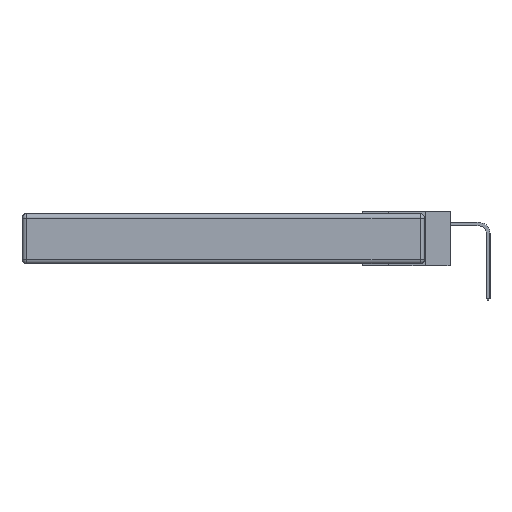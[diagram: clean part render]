
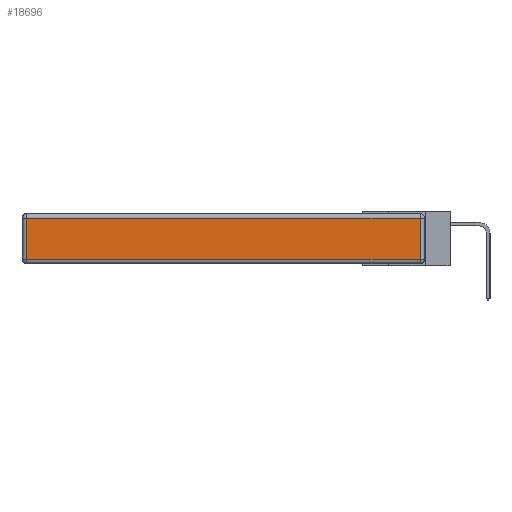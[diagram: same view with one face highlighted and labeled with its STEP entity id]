
A CAD part, left-side view. The second image highlights one B-rep face of the part: STEP entity #18696.
In plain terms, the highlighted planar face has unit normal (-1, 0, 0).
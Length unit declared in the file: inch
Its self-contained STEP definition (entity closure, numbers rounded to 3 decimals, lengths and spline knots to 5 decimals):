
#203 = DIRECTION ( 'NONE',  ( 0., 0., 1. ) ) ;
#385 = CARTESIAN_POINT ( 'NONE',  ( 0., 2.72, -0.343 ) ) ;
#1299 = CARTESIAN_POINT ( 'NONE',  ( 0., 0., -0.313 ) ) ;
#3633 = LINE ( 'NONE', #25424, #27488 ) ;
#4889 = LINE ( 'NONE', #385, #25835 ) ;
#6402 = EDGE_CURVE ( 'NONE', #10515, #11674, #4889, .T. ) ;
#6538 = EDGE_LOOP ( 'NONE', ( #11590, #15237, #15600, #9331 ) ) ;
#8997 = FACE_OUTER_BOUND ( 'NONE', #6538, .T. ) ;
#9331 = ORIENTED_EDGE ( 'NONE', *, *, #6402, .T. ) ;
#10515 = VERTEX_POINT ( 'NONE', #21889 ) ;
#11590 = ORIENTED_EDGE ( 'NONE', *, *, #17142, .T. ) ;
#11674 = VERTEX_POINT ( 'NONE', #11871 ) ;
#11871 = CARTESIAN_POINT ( 'NONE',  ( 0., 2.72, -0.313 ) ) ;
#13286 = CARTESIAN_POINT ( 'NONE',  ( 0., 0.03, -0.313 ) ) ;
#14312 = DIRECTION ( 'NONE',  ( -1., 0., 0. ) ) ;
#15237 = ORIENTED_EDGE ( 'NONE', *, *, #17485, .T. ) ;
#15278 = CARTESIAN_POINT ( 'NONE',  ( 0., 0.03, -0.03 ) ) ;
#15600 = ORIENTED_EDGE ( 'NONE', *, *, #19342, .T. ) ;
#15658 = VERTEX_POINT ( 'NONE', #13286 ) ;
#16502 = DIRECTION ( 'NONE',  ( 0., 0., 1. ) ) ;
#16970 = VECTOR ( 'NONE', #17505, 39.37008 ) ;
#17142 = EDGE_CURVE ( 'NONE', #11674, #15658, #23798, .T. ) ;
#17485 = EDGE_CURVE ( 'NONE', #15658, #26995, #3633, .T. ) ;
#17505 = DIRECTION ( 'NONE',  ( 0., -1., 0. ) ) ;
#18696 = ADVANCED_FACE ( 'NONE', ( #8997 ), #27871, .T. ) ;
#19290 = DIRECTION ( 'NONE',  ( 0., 0., -1. ) ) ;
#19342 = EDGE_CURVE ( 'NONE', #26995, #10515, #23038, .T. ) ;
#21889 = CARTESIAN_POINT ( 'NONE',  ( 0., 2.72, -0.03 ) ) ;
#22449 = DIRECTION ( 'NONE',  ( 0., 1., 0. ) ) ;
#23038 = LINE ( 'NONE', #26998, #28422 ) ;
#23437 = CARTESIAN_POINT ( 'NONE',  ( 0., 0., -0.343 ) ) ;
#23798 = LINE ( 'NONE', #1299, #16970 ) ;
#25424 = CARTESIAN_POINT ( 'NONE',  ( 0., 0.03, -0.343 ) ) ;
#25835 = VECTOR ( 'NONE', #19290, 39.37008 ) ;
#25917 = AXIS2_PLACEMENT_3D ( 'NONE', #23437, #14312, #203 ) ;
#26995 = VERTEX_POINT ( 'NONE', #15278 ) ;
#26998 = CARTESIAN_POINT ( 'NONE',  ( 0., 2.75, -0.03 ) ) ;
#27488 = VECTOR ( 'NONE', #16502, 39.37008 ) ;
#27871 = PLANE ( 'NONE',  #25917 ) ;
#28422 = VECTOR ( 'NONE', #22449, 39.37008 ) ;
